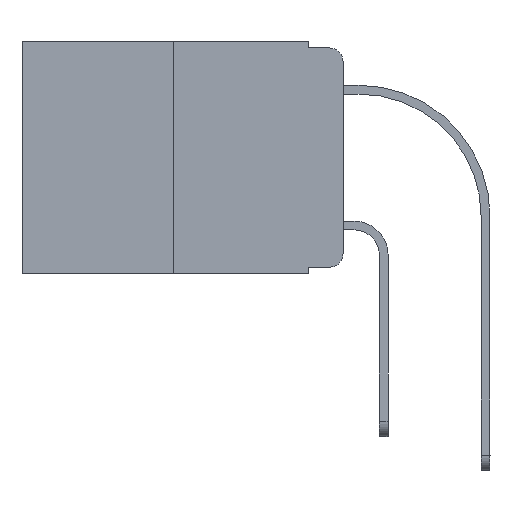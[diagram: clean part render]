
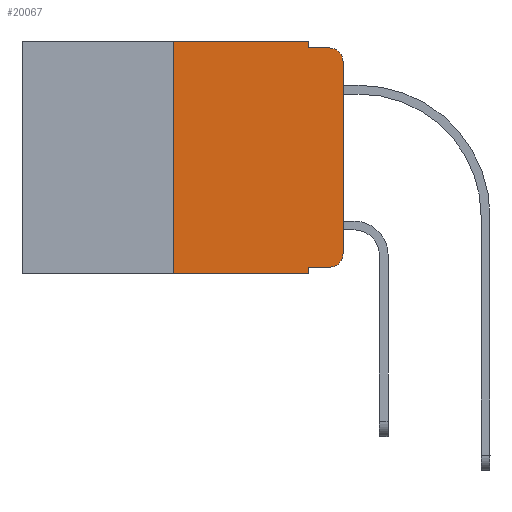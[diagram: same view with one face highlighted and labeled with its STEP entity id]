
A CAD part, left-side view. The second image highlights one B-rep face of the part: STEP entity #20067.
In plain terms, the highlighted planar face has unit normal (-1, 0, 0).
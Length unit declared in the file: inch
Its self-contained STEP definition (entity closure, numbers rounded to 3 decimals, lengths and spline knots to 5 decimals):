
#130 = LINE ( 'NONE', #16178, #20253 ) ;
#375 = EDGE_CURVE ( 'NONE', #1408, #10633, #16431, .T. ) ;
#1088 = DIRECTION ( 'NONE',  ( 0., 0., -1. ) ) ;
#1107 = DIRECTION ( 'NONE',  ( 0., 0., 1. ) ) ;
#1408 = VERTEX_POINT ( 'NONE', #5816 ) ;
#1782 = DIRECTION ( 'NONE',  ( 0., -1., 0. ) ) ;
#2187 = DIRECTION ( 'NONE',  ( 0., 0., 1. ) ) ;
#2469 = CARTESIAN_POINT ( 'NONE',  ( 0., 0.02, -0.313 ) ) ;
#2803 = ORIENTED_EDGE ( 'NONE', *, *, #22378, .F. ) ;
#3768 = CARTESIAN_POINT ( 'NONE',  ( 0., 0.473, -0.343 ) ) ;
#3832 = VERTEX_POINT ( 'NONE', #21274 ) ;
#4049 = LINE ( 'NONE', #12020, #16977 ) ;
#4564 = DIRECTION ( 'NONE',  ( 1., 0., 0. ) ) ;
#4731 = DIRECTION ( 'NONE',  ( -1., 0., 0. ) ) ;
#5816 = CARTESIAN_POINT ( 'NONE',  ( 0., 0., -0.03 ) ) ;
#5865 = VERTEX_POINT ( 'NONE', #21329 ) ;
#6521 = CIRCLE ( 'NONE', #14571, 0.02 ) ;
#6944 = EDGE_CURVE ( 'NONE', #10801, #3832, #14182, .T. ) ;
#6977 = CARTESIAN_POINT ( 'NONE',  ( 0., 0.051, -0.343 ) ) ;
#7818 = EDGE_CURVE ( 'NONE', #5865, #8893, #21959, .T. ) ;
#8224 = DIRECTION ( 'NONE',  ( 0., 0., -1. ) ) ;
#8675 = ORIENTED_EDGE ( 'NONE', *, *, #25225, .T. ) ;
#8814 = AXIS2_PLACEMENT_3D ( 'NONE', #13284, #13146, #1088 ) ;
#8893 = VERTEX_POINT ( 'NONE', #6977 ) ;
#8930 = VERTEX_POINT ( 'NONE', #19433 ) ;
#9331 = LINE ( 'NONE', #9873, #9541 ) ;
#9541 = VECTOR ( 'NONE', #25529, 39.37008 ) ;
#9873 = CARTESIAN_POINT ( 'NONE',  ( 0., 0.051, 0. ) ) ;
#10166 = FACE_OUTER_BOUND ( 'NONE', #10950, .T. ) ;
#10633 = VERTEX_POINT ( 'NONE', #11992 ) ;
#10657 = ORIENTED_EDGE ( 'NONE', *, *, #16324, .T. ) ;
#10801 = VERTEX_POINT ( 'NONE', #16617 ) ;
#10950 = EDGE_LOOP ( 'NONE', ( #8675, #16059, #2803, #25396, #22877, #20338, #23787, #20838, #24752, #10657 ) ) ;
#11470 = LINE ( 'NONE', #26065, #17045 ) ;
#11564 = VECTOR ( 'NONE', #1782, 39.37008 ) ;
#11823 = LINE ( 'NONE', #20310, #19739 ) ;
#11881 = EDGE_CURVE ( 'NONE', #21133, #13529, #9331, .T. ) ;
#11992 = CARTESIAN_POINT ( 'NONE',  ( 0., 0.02, -0.01 ) ) ;
#12020 = CARTESIAN_POINT ( 'NONE',  ( 0., 0.25, 0. ) ) ;
#12368 = EDGE_CURVE ( 'NONE', #21996, #21133, #11823, .T. ) ;
#12453 = DIRECTION ( 'NONE',  ( 0., 0., -1. ) ) ;
#13146 = DIRECTION ( 'NONE',  ( -1., 0., 0. ) ) ;
#13284 = CARTESIAN_POINT ( 'NONE',  ( 0., 0.02, -0.03 ) ) ;
#13529 = VERTEX_POINT ( 'NONE', #17842 ) ;
#13534 = EDGE_CURVE ( 'NONE', #5865, #21996, #4049, .T. ) ;
#14182 = LINE ( 'NONE', #24004, #16171 ) ;
#14337 = DIRECTION ( 'NONE',  ( 0., -1., 0. ) ) ;
#14571 = AXIS2_PLACEMENT_3D ( 'NONE', #2469, #4731, #12453 ) ;
#15139 = VECTOR ( 'NONE', #1107, 39.37008 ) ;
#15599 = CARTESIAN_POINT ( 'NONE',  ( 0., 0.473, 0. ) ) ;
#16059 = ORIENTED_EDGE ( 'NONE', *, *, #375, .T. ) ;
#16171 = VECTOR ( 'NONE', #22281, 39.37008 ) ;
#16178 = CARTESIAN_POINT ( 'NONE',  ( 0., 0.051, 0. ) ) ;
#16324 = EDGE_CURVE ( 'NONE', #3832, #8930, #6521, .T. ) ;
#16431 = CIRCLE ( 'NONE', #8814, 0.02 ) ;
#16617 = CARTESIAN_POINT ( 'NONE',  ( 0., 0.051, -0.333 ) ) ;
#16977 = VECTOR ( 'NONE', #2187, 39.37008 ) ;
#17045 = VECTOR ( 'NONE', #17566, 39.37008 ) ;
#17566 = DIRECTION ( 'NONE',  ( 0., -1., 0. ) ) ;
#17842 = CARTESIAN_POINT ( 'NONE',  ( 0., 0.051, -0.01 ) ) ;
#19284 = LINE ( 'NONE', #23405, #15139 ) ;
#19433 = CARTESIAN_POINT ( 'NONE',  ( 0., 0., -0.313 ) ) ;
#19733 = CARTESIAN_POINT ( 'NONE',  ( 0., 0.25, 0. ) ) ;
#19739 = VECTOR ( 'NONE', #14337, 39.37008 ) ;
#20067 = ADVANCED_FACE ( 'NONE', ( #10166 ), #25685, .F. ) ;
#20253 = VECTOR ( 'NONE', #8224, 39.37008 ) ;
#20310 = CARTESIAN_POINT ( 'NONE',  ( 0., 0.473, 0. ) ) ;
#20338 = ORIENTED_EDGE ( 'NONE', *, *, #13534, .F. ) ;
#20838 = ORIENTED_EDGE ( 'NONE', *, *, #26005, .F. ) ;
#21133 = VERTEX_POINT ( 'NONE', #23708 ) ;
#21274 = CARTESIAN_POINT ( 'NONE',  ( 0., 0.02, -0.333 ) ) ;
#21329 = CARTESIAN_POINT ( 'NONE',  ( 0., 0.25, -0.343 ) ) ;
#21959 = LINE ( 'NONE', #3768, #11564 ) ;
#21996 = VERTEX_POINT ( 'NONE', #19733 ) ;
#22281 = DIRECTION ( 'NONE',  ( 0., -1., 0. ) ) ;
#22378 = EDGE_CURVE ( 'NONE', #13529, #10633, #11470, .T. ) ;
#22761 = DIRECTION ( 'NONE',  ( 0., 0., -1. ) ) ;
#22877 = ORIENTED_EDGE ( 'NONE', *, *, #12368, .F. ) ;
#23365 = AXIS2_PLACEMENT_3D ( 'NONE', #15599, #4564, #22761 ) ;
#23405 = CARTESIAN_POINT ( 'NONE',  ( 0., 0., 0. ) ) ;
#23708 = CARTESIAN_POINT ( 'NONE',  ( 0., 0.051, 0. ) ) ;
#23787 = ORIENTED_EDGE ( 'NONE', *, *, #7818, .T. ) ;
#24004 = CARTESIAN_POINT ( 'NONE',  ( 0., 0.051, -0.333 ) ) ;
#24752 = ORIENTED_EDGE ( 'NONE', *, *, #6944, .T. ) ;
#25225 = EDGE_CURVE ( 'NONE', #8930, #1408, #19284, .T. ) ;
#25396 = ORIENTED_EDGE ( 'NONE', *, *, #11881, .F. ) ;
#25529 = DIRECTION ( 'NONE',  ( 0., 0., -1. ) ) ;
#25685 = PLANE ( 'NONE',  #23365 ) ;
#26005 = EDGE_CURVE ( 'NONE', #10801, #8893, #130, .T. ) ;
#26065 = CARTESIAN_POINT ( 'NONE',  ( 0., 0.051, -0.01 ) ) ;
